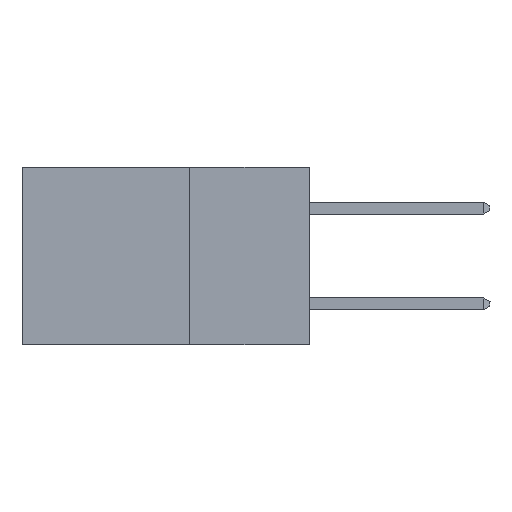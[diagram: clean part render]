
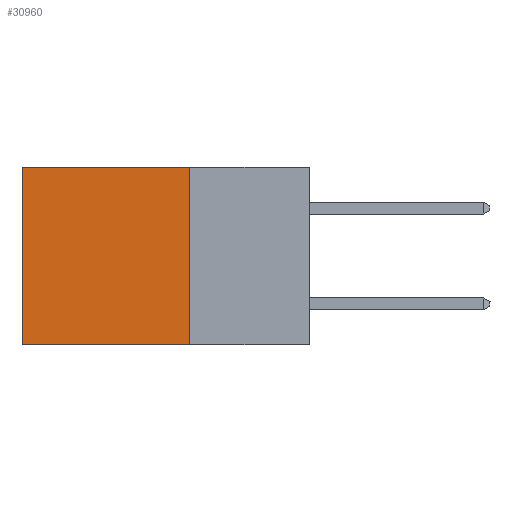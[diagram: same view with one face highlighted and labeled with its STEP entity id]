
A CAD part, left-side view. The second image highlights one B-rep face of the part: STEP entity #30960.
In plain terms, the highlighted planar face has unit normal (-1, 0, 0).
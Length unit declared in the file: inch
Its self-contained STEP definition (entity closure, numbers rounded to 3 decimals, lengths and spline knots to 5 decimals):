
#1618 = ORIENTED_EDGE ( 'NONE', *, *, #32017, .F. ) ;
#1950 = CARTESIAN_POINT ( 'NONE',  ( 0.2875, 0.25, -0.37 ) ) ;
#2495 = DIRECTION ( 'NONE',  ( 0., 0., -1. ) ) ;
#3412 = VECTOR ( 'NONE', #23747, 39.37008 ) ;
#4969 = DIRECTION ( 'NONE',  ( 0., 1., 0. ) ) ;
#5136 = ORIENTED_EDGE ( 'NONE', *, *, #10785, .T. ) ;
#5434 = VERTEX_POINT ( 'NONE', #24606 ) ;
#6771 = CARTESIAN_POINT ( 'NONE',  ( 0.2875, 0.6, 0. ) ) ;
#9465 = PLANE ( 'NONE',  #36017 ) ;
#10785 = EDGE_CURVE ( 'NONE', #20437, #42258, #33143, .T. ) ;
#11117 = CARTESIAN_POINT ( 'NONE',  ( 0.2875, 0.25, 0. ) ) ;
#13935 = CARTESIAN_POINT ( 'NONE',  ( 0.2875, 0.25, 0. ) ) ;
#15190 = CARTESIAN_POINT ( 'NONE',  ( 0.2875, 0.25, 0. ) ) ;
#17389 = LINE ( 'NONE', #13935, #3412 ) ;
#17672 = FACE_OUTER_BOUND ( 'NONE', #23633, .T. ) ;
#18856 = VECTOR ( 'NONE', #19917, 39.37008 ) ;
#18961 = DIRECTION ( 'NONE',  ( 1., 0., 0. ) ) ;
#19878 = VERTEX_POINT ( 'NONE', #42661 ) ;
#19917 = DIRECTION ( 'NONE',  ( 0., 0., -1. ) ) ;
#20437 = VERTEX_POINT ( 'NONE', #15190 ) ;
#23078 = ORIENTED_EDGE ( 'NONE', *, *, #28609, .T. ) ;
#23284 = LINE ( 'NONE', #1950, #24320 ) ;
#23633 = EDGE_LOOP ( 'NONE', ( #23078, #1618, #42737, #5136 ) ) ;
#23747 = DIRECTION ( 'NONE',  ( 0., 0., -1. ) ) ;
#24320 = VECTOR ( 'NONE', #4969, 39.37008 ) ;
#24606 = CARTESIAN_POINT ( 'NONE',  ( 0.2875, 0.25, -0.37 ) ) ;
#27815 = DIRECTION ( 'NONE',  ( 0., 1., 0. ) ) ;
#28609 = EDGE_CURVE ( 'NONE', #42258, #19878, #30753, .T. ) ;
#29665 = CARTESIAN_POINT ( 'NONE',  ( 0.2875, 0.6, 0. ) ) ;
#30753 = LINE ( 'NONE', #6771, #18856 ) ;
#30960 = ADVANCED_FACE ( 'NONE', ( #17672 ), #9465, .F. ) ;
#32017 = EDGE_CURVE ( 'NONE', #5434, #19878, #23284, .T. ) ;
#33143 = LINE ( 'NONE', #11117, #39375 ) ;
#35463 = EDGE_CURVE ( 'NONE', #20437, #5434, #17389, .T. ) ;
#36017 = AXIS2_PLACEMENT_3D ( 'NONE', #42501, #18961, #2495 ) ;
#39375 = VECTOR ( 'NONE', #27815, 39.37008 ) ;
#42258 = VERTEX_POINT ( 'NONE', #29665 ) ;
#42501 = CARTESIAN_POINT ( 'NONE',  ( 0.2875, 0.25, 0. ) ) ;
#42661 = CARTESIAN_POINT ( 'NONE',  ( 0.2875, 0.6, -0.37 ) ) ;
#42737 = ORIENTED_EDGE ( 'NONE', *, *, #35463, .F. ) ;
